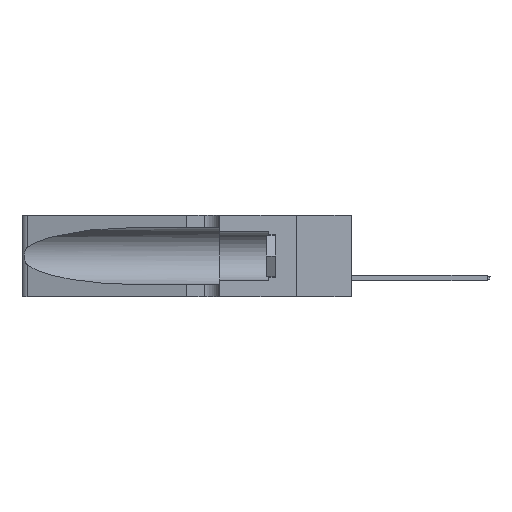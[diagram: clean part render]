
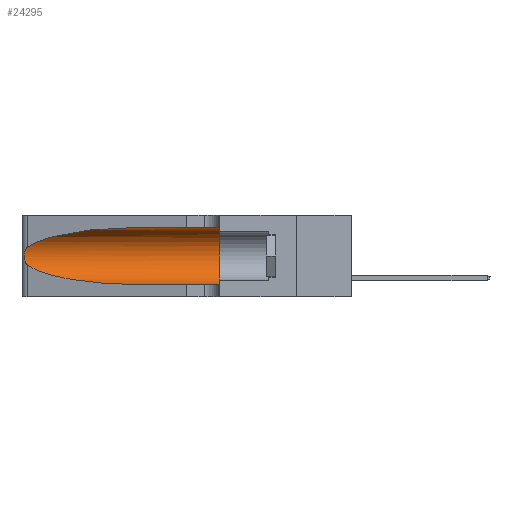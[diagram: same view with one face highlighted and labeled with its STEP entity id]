
A CAD part, left-side view. The second image highlights one B-rep face of the part: STEP entity #24295.
In plain terms, the highlighted cylindrical face has radius 3.308 mm (diameter 6.617 mm), a partial arc.
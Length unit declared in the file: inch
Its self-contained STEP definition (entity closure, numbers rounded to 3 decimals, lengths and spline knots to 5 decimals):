
#26 = CARTESIAN_POINT ( 'NONE',  ( 0.2373, 1.15595, 0.08982 ) ) ;
#69 = CARTESIAN_POINT ( 'NONE',  ( 0.1305, 0.72297, 0.05475 ) ) ;
#275 = DIRECTION ( 'NONE',  ( 0., -1., 0. ) ) ;
#616 = CARTESIAN_POINT ( 'NONE',  ( 0.25487, 1.22718, 0.22369 ) ) ;
#831 =( BOUNDED_CURVE ( )  B_SPLINE_CURVE ( 3, ( #4686, #6536, #4772, #20823 ),
 .UNSPECIFIED., .F., .F. ) 
 B_SPLINE_CURVE_WITH_KNOTS ( ( 4, 4 ),
 ( 1.5708, 2.84003 ),
 .UNSPECIFIED. ) 
 CURVE ( )  GEOMETRIC_REPRESENTATION_ITEM ( )  RATIONAL_B_SPLINE_CURVE ( ( 1., 0.87, 0.87, 1. ) ) 
 REPRESENTATION_ITEM ( '' )  );
#1115 = VECTOR ( 'NONE', #14464, 39.37008 ) ;
#1169 = CARTESIAN_POINT ( 'NONE',  ( 0.25639, 1.23186, 0.15144 ) ) ;
#1847 = CARTESIAN_POINT ( 'NONE',  ( 0.25639, 1.23184, 0.21858 ) ) ;
#3233 = EDGE_CURVE ( 'NONE', #25388, #6565, #5166, .T. ) ;
#3461 = CARTESIAN_POINT ( 'NONE',  ( 0.25555, 1.22993, 0.14849 ) ) ;
#3839 = DIRECTION ( 'NONE',  ( 0., 1., 0. ) ) ;
#3949 = FACE_OUTER_BOUND ( 'NONE', #16903, .T. ) ;
#4686 = CARTESIAN_POINT ( 'NONE',  ( 0.1305, 0.72297, 0.31525 ) ) ;
#4772 = CARTESIAN_POINT ( 'NONE',  ( 0.2373, 1.15595, 0.28018 ) ) ;
#4856 = VECTOR ( 'NONE', #17621, 39.37008 ) ;
#4999 = CARTESIAN_POINT ( 'NONE',  ( 0.1305, 0.35, 0.31525 ) ) ;
#5011 = EDGE_CURVE ( 'NONE', #19339, #25388, #18133, .T. ) ;
#5095 = EDGE_CURVE ( 'NONE', #12078, #19339, #16198, .T. ) ;
#5166 = LINE ( 'NONE', #15277, #4856 ) ;
#5752 = VERTEX_POINT ( 'NONE', #4999 ) ;
#5975 = CARTESIAN_POINT ( 'NONE',  ( 0.26018, 1.23835, 0.19895 ) ) ;
#6536 = CARTESIAN_POINT ( 'NONE',  ( 0.18966, 0.96281, 0.31525 ) ) ;
#6565 = VERTEX_POINT ( 'NONE', #14109 ) ;
#6765 = CYLINDRICAL_SURFACE ( 'NONE', #19647, 0.13025 ) ;
#7232 = CARTESIAN_POINT ( 'NONE',  ( 0.25487, 1.22718, 0.22369 ) ) ;
#7910 = CARTESIAN_POINT ( 'NONE',  ( 0.1305, 0.35, 0.185 ) ) ;
#8113 = DIRECTION ( 'NONE',  ( 0., 0., -1. ) ) ;
#8401 = CARTESIAN_POINT ( 'NONE',  ( 0.1305, 1.61858, 0.31525 ) ) ;
#8628 = CARTESIAN_POINT ( 'NONE',  ( 0.25854, 1.2359, 0.20912 ) ) ;
#10154 = CARTESIAN_POINT ( 'NONE',  ( 0.1305, 1.61858, 0.185 ) ) ;
#10408 = ORIENTED_EDGE ( 'NONE', *, *, #3233, .T. ) ;
#10660 = ORIENTED_EDGE ( 'NONE', *, *, #21655, .F. ) ;
#10724 = CARTESIAN_POINT ( 'NONE',  ( 0.26017, 1.23833, 0.17102 ) ) ;
#11443 = EDGE_CURVE ( 'NONE', #24526, #12078, #831, .T. ) ;
#12078 = VERTEX_POINT ( 'NONE', #616 ) ;
#12233 = ORIENTED_EDGE ( 'NONE', *, *, #5095, .T. ) ;
#12356 = AXIS2_PLACEMENT_3D ( 'NONE', #7910, #3839, #17993 ) ;
#12637 = CARTESIAN_POINT ( 'NONE',  ( 0.25787, 1.23484, 0.2124 ) ) ;
#13075 = CARTESIAN_POINT ( 'NONE',  ( 0.26075, 1.23896, 0.19203 ) ) ;
#13292 = CARTESIAN_POINT ( 'NONE',  ( 0.25487, 1.22718, 0.14631 ) ) ;
#13565 = ORIENTED_EDGE ( 'NONE', *, *, #11443, .T. ) ;
#13597 = CARTESIAN_POINT ( 'NONE',  ( 0.25487, 1.22718, 0.14631 ) ) ;
#14109 = CARTESIAN_POINT ( 'NONE',  ( 0.1305, 0.35, 0.05475 ) ) ;
#14464 = DIRECTION ( 'NONE',  ( 0., -1., 0. ) ) ;
#15277 = CARTESIAN_POINT ( 'NONE',  ( 0.1305, 1.61858, 0.05475 ) ) ;
#15523 = CIRCLE ( 'NONE', #12356, 0.13025 ) ;
#16198 = B_SPLINE_CURVE_WITH_KNOTS ( 'NONE', 3,
 ( #7232, #24887, #1847, #12637, #8628, #5975, #13075, #19899, #10724, #17351, #25198, #1169, #3461, #13597 ),
 .UNSPECIFIED., .F., .F.,
 ( 4, 2, 2, 2, 2, 2, 4 ),
 ( 0., 0.00027, 0.00053, 0.00107, 0.0016, 0.00187, 0.00214 ),
 .UNSPECIFIED. ) ;
#16903 = EDGE_LOOP ( 'NONE', ( #13565, #12233, #20558, #10408, #10660, #20434 ) ) ;
#17351 = CARTESIAN_POINT ( 'NONE',  ( 0.25856, 1.23593, 0.16098 ) ) ;
#17621 = DIRECTION ( 'NONE',  ( 0., -1., 0. ) ) ;
#17993 = DIRECTION ( 'NONE',  ( 0., 0., 1. ) ) ;
#18133 =( BOUNDED_CURVE ( )  B_SPLINE_CURVE ( 3, ( #22222, #26, #24253, #26307 ),
 .UNSPECIFIED., .F., .F. ) 
 B_SPLINE_CURVE_WITH_KNOTS ( ( 4, 4 ),
 ( 3.44316, 4.71239 ),
 .UNSPECIFIED. ) 
 CURVE ( )  GEOMETRIC_REPRESENTATION_ITEM ( )  RATIONAL_B_SPLINE_CURVE ( ( 1., 0.87, 0.87, 1. ) ) 
 REPRESENTATION_ITEM ( '' )  );
#19339 = VERTEX_POINT ( 'NONE', #13292 ) ;
#19647 = AXIS2_PLACEMENT_3D ( 'NONE', #10154, #275, #8113 ) ;
#19899 = CARTESIAN_POINT ( 'NONE',  ( 0.26075, 1.23896, 0.178 ) ) ;
#20434 = ORIENTED_EDGE ( 'NONE', *, *, #23796, .F. ) ;
#20558 = ORIENTED_EDGE ( 'NONE', *, *, #5011, .T. ) ;
#20823 = CARTESIAN_POINT ( 'NONE',  ( 0.25487, 1.22718, 0.22369 ) ) ;
#21655 = EDGE_CURVE ( 'NONE', #5752, #6565, #15523, .T. ) ;
#22222 = CARTESIAN_POINT ( 'NONE',  ( 0.25487, 1.22718, 0.14631 ) ) ;
#23353 = CARTESIAN_POINT ( 'NONE',  ( 0.1305, 0.72297, 0.31525 ) ) ;
#23796 = EDGE_CURVE ( 'NONE', #24526, #5752, #25966, .T. ) ;
#24253 = CARTESIAN_POINT ( 'NONE',  ( 0.18966, 0.96281, 0.05475 ) ) ;
#24295 = ADVANCED_FACE ( 'NONE', ( #3949 ), #6765, .F. ) ;
#24526 = VERTEX_POINT ( 'NONE', #23353 ) ;
#24887 = CARTESIAN_POINT ( 'NONE',  ( 0.25555, 1.22994, 0.2215 ) ) ;
#25198 = CARTESIAN_POINT ( 'NONE',  ( 0.25789, 1.23486, 0.15765 ) ) ;
#25388 = VERTEX_POINT ( 'NONE', #69 ) ;
#25966 = LINE ( 'NONE', #8401, #1115 ) ;
#26307 = CARTESIAN_POINT ( 'NONE',  ( 0.1305, 0.72297, 0.05475 ) ) ;
